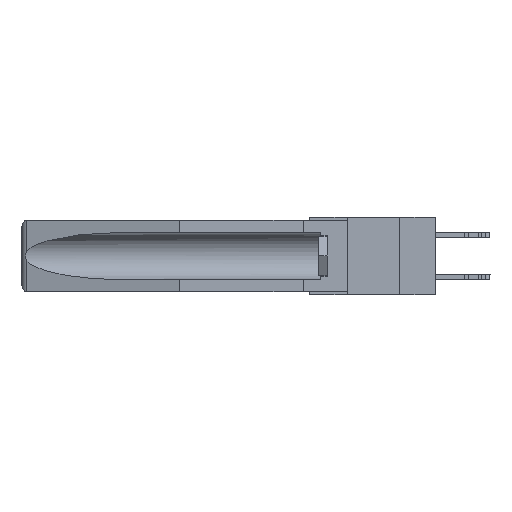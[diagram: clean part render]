
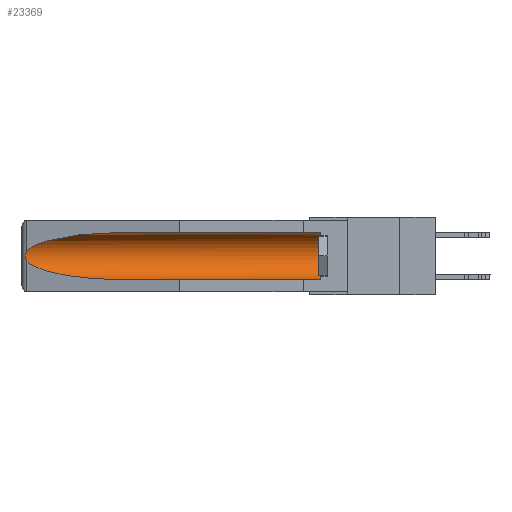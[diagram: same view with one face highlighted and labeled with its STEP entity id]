
A CAD part, left-side view. The second image highlights one B-rep face of the part: STEP entity #23369.
In plain terms, the highlighted cylindrical face has radius 2.857 mm (diameter 5.715 mm), a partial arc.
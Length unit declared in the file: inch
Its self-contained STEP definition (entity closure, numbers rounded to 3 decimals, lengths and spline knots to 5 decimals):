
#61 = VERTEX_POINT ( 'NONE', #7413 ) ;
#510 = CIRCLE ( 'NONE', #21991, 0.1125 ) ;
#736 = CARTESIAN_POINT ( 'NONE',  ( 0.26537, 1.52718, -0.19328 ) ) ;
#1003 = CARTESIAN_POINT ( 'NONE',  ( 0.26654, 1.53092, -0.15636 ) ) ;
#1018 = VERTEX_POINT ( 'NONE', #33407 ) ;
#1229 = EDGE_CURVE ( 'NONE', #11696, #20214, #7290, .T. ) ;
#1584 = CARTESIAN_POINT ( 'NONE',  ( 0.2675, 1.53308, -0.17534 ) ) ;
#2940 = EDGE_LOOP ( 'NONE', ( #5318, #25567, #17268, #4884, #23923, #12337 ) ) ;
#3071 = DIRECTION ( 'NONE',  ( 0., 0., 1. ) ) ;
#4243 = CARTESIAN_POINT ( 'NONE',  ( 0.26597, 1.5296, -0.19026 ) ) ;
#4665 = CARTESIAN_POINT ( 'NONE',  ( 0.26537, 1.52718, -0.14972 ) ) ;
#4884 = ORIENTED_EDGE ( 'NONE', *, *, #27279, .F. ) ;
#5036 = CARTESIAN_POINT ( 'NONE',  ( 0.26537, 1.52718, -0.14972 ) ) ;
#5093 = DIRECTION ( 'NONE',  ( 0., 1., 0. ) ) ;
#5318 = ORIENTED_EDGE ( 'NONE', *, *, #32723, .T. ) ;
#7067 = CARTESIAN_POINT ( 'NONE',  ( 0.26537, 1.52718, -0.19328 ) ) ;
#7260 = CARTESIAN_POINT ( 'NONE',  ( 0.155, 1.07973, -0.059 ) ) ;
#7290 = B_SPLINE_CURVE_WITH_KNOTS ( 'NONE', 3,
 ( #27510, #16925, #1003, #27840, #17524, #1584, #11908, #14674, #4243, #7067 ),
 .UNSPECIFIED., .F., .F.,
 ( 4, 2, 2, 2, 4 ),
 ( 0., 0.00029, 0.00058, 0.00087, 0.00117 ),
 .UNSPECIFIED. ) ;
#7374 = CARTESIAN_POINT ( 'NONE',  ( 0.155, 1.07973, -0.059 ) ) ;
#7413 = CARTESIAN_POINT ( 'NONE',  ( 0.155, 0.126, -0.059 ) ) ;
#9620 = VECTOR ( 'NONE', #5093, 39.37008 ) ;
#9899 = CARTESIAN_POINT ( 'NONE',  ( 0.21114, 1.30732, -0.059 ) ) ;
#10340 = EDGE_CURVE ( 'NONE', #61, #17422, #29173, .T. ) ;
#10970 = DIRECTION ( 'NONE',  ( 0., 1., 0. ) ) ;
#11614 = CARTESIAN_POINT ( 'NONE',  ( 0.155, 1.07973, -0.284 ) ) ;
#11696 = VERTEX_POINT ( 'NONE', #5036 ) ;
#11908 = CARTESIAN_POINT ( 'NONE',  ( 0.2673, 1.53269, -0.17917 ) ) ;
#12337 = ORIENTED_EDGE ( 'NONE', *, *, #10340, .T. ) ;
#13610 = CARTESIAN_POINT ( 'NONE',  ( 0.155, 0.126, -0.1715 ) ) ;
#13745 = VECTOR ( 'NONE', #29551, 39.37008 ) ;
#14424 = EDGE_CURVE ( 'NONE', #1018, #61, #510, .T. ) ;
#14674 = CARTESIAN_POINT ( 'NONE',  ( 0.26655, 1.53094, -0.18657 ) ) ;
#16925 = CARTESIAN_POINT ( 'NONE',  ( 0.26597, 1.52961, -0.15275 ) ) ;
#17268 = ORIENTED_EDGE ( 'NONE', *, *, #17309, .T. ) ;
#17309 = EDGE_CURVE ( 'NONE', #20214, #22001, #19224, .T. ) ;
#17422 = VERTEX_POINT ( 'NONE', #7374 ) ;
#17524 = CARTESIAN_POINT ( 'NONE',  ( 0.2675, 1.53308, -0.16763 ) ) ;
#19100 = CARTESIAN_POINT ( 'NONE',  ( 0.155, -0.30754, -0.059 ) ) ;
#19224 =( BOUNDED_CURVE ( )  B_SPLINE_CURVE ( 3, ( #34085, #33975, #31041, #23304 ),
 .UNSPECIFIED., .F., .F. ) 
 B_SPLINE_CURVE_WITH_KNOTS ( ( 4, 4 ),
 ( 0.1948, 1.5708 ),
 .UNSPECIFIED. ) 
 CURVE ( )  GEOMETRIC_REPRESENTATION_ITEM ( )  RATIONAL_B_SPLINE_CURVE ( ( 1., 0.848, 0.848, 1. ) ) 
 REPRESENTATION_ITEM ( '' )  );
#20214 = VERTEX_POINT ( 'NONE', #736 ) ;
#20642 = CARTESIAN_POINT ( 'NONE',  ( 0.25451, 1.48313, -0.09465 ) ) ;
#20912 = LINE ( 'NONE', #29445, #13745 ) ;
#21991 = AXIS2_PLACEMENT_3D ( 'NONE', #13610, #32613, #3071 ) ;
#22001 = VERTEX_POINT ( 'NONE', #11614 ) ;
#23304 = CARTESIAN_POINT ( 'NONE',  ( 0.155, 1.07973, -0.284 ) ) ;
#23369 = ADVANCED_FACE ( 'NONE', ( #34247 ), #24290, .F. ) ;
#23923 = ORIENTED_EDGE ( 'NONE', *, *, #14424, .T. ) ;
#24290 = CYLINDRICAL_SURFACE ( 'NONE', #29669, 0.1125 ) ;
#25567 = ORIENTED_EDGE ( 'NONE', *, *, #1229, .T. ) ;
#26817 = CARTESIAN_POINT ( 'NONE',  ( 0.155, -0.30754, -0.1715 ) ) ;
#27279 = EDGE_CURVE ( 'NONE', #1018, #22001, #20912, .T. ) ;
#27510 = CARTESIAN_POINT ( 'NONE',  ( 0.26537, 1.52718, -0.14972 ) ) ;
#27840 = CARTESIAN_POINT ( 'NONE',  ( 0.2673, 1.5327, -0.16383 ) ) ;
#29173 = LINE ( 'NONE', #19100, #9620 ) ;
#29445 = CARTESIAN_POINT ( 'NONE',  ( 0.155, -0.30754, -0.284 ) ) ;
#29551 = DIRECTION ( 'NONE',  ( 0., 1., 0. ) ) ;
#29669 = AXIS2_PLACEMENT_3D ( 'NONE', #26817, #10970, #32273 ) ;
#31014 =( BOUNDED_CURVE ( )  B_SPLINE_CURVE ( 3, ( #7260, #9899, #20642, #4665 ),
 .UNSPECIFIED., .F., .F. ) 
 B_SPLINE_CURVE_WITH_KNOTS ( ( 4, 4 ),
 ( 4.71239, 6.08839 ),
 .UNSPECIFIED. ) 
 CURVE ( )  GEOMETRIC_REPRESENTATION_ITEM ( )  RATIONAL_B_SPLINE_CURVE ( ( 1., 0.848, 0.848, 1. ) ) 
 REPRESENTATION_ITEM ( '' )  );
#31041 = CARTESIAN_POINT ( 'NONE',  ( 0.21114, 1.30732, -0.284 ) ) ;
#32273 = DIRECTION ( 'NONE',  ( 0., 0., 1. ) ) ;
#32613 = DIRECTION ( 'NONE',  ( 0., -1., 0. ) ) ;
#32723 = EDGE_CURVE ( 'NONE', #17422, #11696, #31014, .T. ) ;
#33407 = CARTESIAN_POINT ( 'NONE',  ( 0.155, 0.126, -0.284 ) ) ;
#33975 = CARTESIAN_POINT ( 'NONE',  ( 0.25451, 1.48313, -0.24835 ) ) ;
#34085 = CARTESIAN_POINT ( 'NONE',  ( 0.26537, 1.52718, -0.19328 ) ) ;
#34247 = FACE_OUTER_BOUND ( 'NONE', #2940, .T. ) ;
